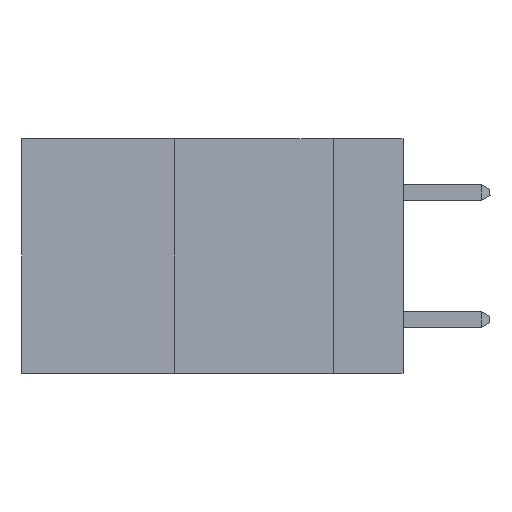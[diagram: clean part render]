
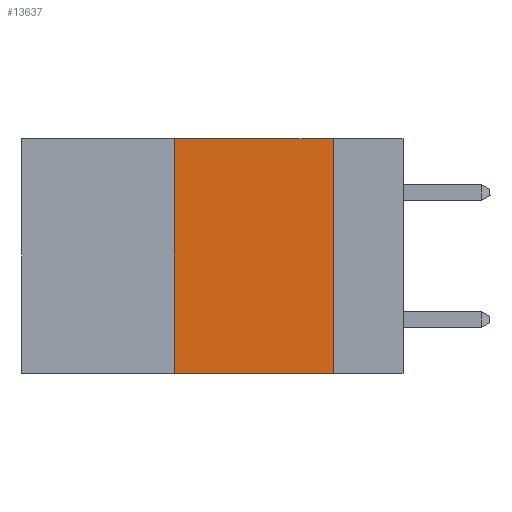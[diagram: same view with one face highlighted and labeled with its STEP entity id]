
A CAD part, left-side view. The second image highlights one B-rep face of the part: STEP entity #13637.
In plain terms, the highlighted planar face has unit normal (-1, 0, 0).
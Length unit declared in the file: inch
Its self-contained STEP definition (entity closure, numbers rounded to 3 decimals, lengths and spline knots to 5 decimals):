
#619 = VERTEX_POINT ( 'NONE', #14502 ) ;
#1363 = DIRECTION ( 'NONE',  ( 0., -1., 0. ) ) ;
#1595 = DIRECTION ( 'NONE',  ( 0., 0., -1. ) ) ;
#2914 = LINE ( 'NONE', #5732, #4387 ) ;
#3286 = EDGE_CURVE ( 'NONE', #12672, #9602, #2914, .T. ) ;
#3331 = CARTESIAN_POINT ( 'NONE',  ( 0., 0.11, -0.37 ) ) ;
#3788 = ORIENTED_EDGE ( 'NONE', *, *, #3286, .F. ) ;
#4278 = ORIENTED_EDGE ( 'NONE', *, *, #11910, .T. ) ;
#4387 = VECTOR ( 'NONE', #5822, 39.37008 ) ;
#4505 = CARTESIAN_POINT ( 'NONE',  ( 0., 0.6, 0. ) ) ;
#4568 = CARTESIAN_POINT ( 'NONE',  ( 0., 0.6, -0.37 ) ) ;
#5543 = EDGE_LOOP ( 'NONE', ( #3788, #16100, #8153, #4278 ) ) ;
#5732 = CARTESIAN_POINT ( 'NONE',  ( 0., 0.11, 0. ) ) ;
#5822 = DIRECTION ( 'NONE',  ( 0., 0., -1. ) ) ;
#5922 = LINE ( 'NONE', #4568, #6996 ) ;
#6166 = EDGE_CURVE ( 'NONE', #619, #12672, #12425, .T. ) ;
#6564 = DIRECTION ( 'NONE',  ( 0., 0., 1. ) ) ;
#6645 = LINE ( 'NONE', #13485, #14883 ) ;
#6753 = AXIS2_PLACEMENT_3D ( 'NONE', #4505, #12482, #1595 ) ;
#6996 = VECTOR ( 'NONE', #14370, 39.37008 ) ;
#7310 = VERTEX_POINT ( 'NONE', #10530 ) ;
#8153 = ORIENTED_EDGE ( 'NONE', *, *, #13862, .F. ) ;
#8489 = PLANE ( 'NONE',  #6753 ) ;
#9602 = VERTEX_POINT ( 'NONE', #3331 ) ;
#10530 = CARTESIAN_POINT ( 'NONE',  ( 0., 0.36, -0.37 ) ) ;
#10968 = CARTESIAN_POINT ( 'NONE',  ( 0., 0.6, 0. ) ) ;
#11910 = EDGE_CURVE ( 'NONE', #7310, #9602, #5922, .T. ) ;
#12066 = CARTESIAN_POINT ( 'NONE',  ( 0., 0.11, 0. ) ) ;
#12177 = VECTOR ( 'NONE', #1363, 39.37008 ) ;
#12425 = LINE ( 'NONE', #10968, #12177 ) ;
#12482 = DIRECTION ( 'NONE',  ( 1., 0., 0. ) ) ;
#12576 = FACE_OUTER_BOUND ( 'NONE', #5543, .T. ) ;
#12672 = VERTEX_POINT ( 'NONE', #12066 ) ;
#13485 = CARTESIAN_POINT ( 'NONE',  ( 0., 0.36, 0. ) ) ;
#13637 = ADVANCED_FACE ( 'NONE', ( #12576 ), #8489, .F. ) ;
#13862 = EDGE_CURVE ( 'NONE', #7310, #619, #6645, .T. ) ;
#14370 = DIRECTION ( 'NONE',  ( 0., -1., 0. ) ) ;
#14502 = CARTESIAN_POINT ( 'NONE',  ( 0., 0.36, 0. ) ) ;
#14883 = VECTOR ( 'NONE', #6564, 39.37008 ) ;
#16100 = ORIENTED_EDGE ( 'NONE', *, *, #6166, .F. ) ;
